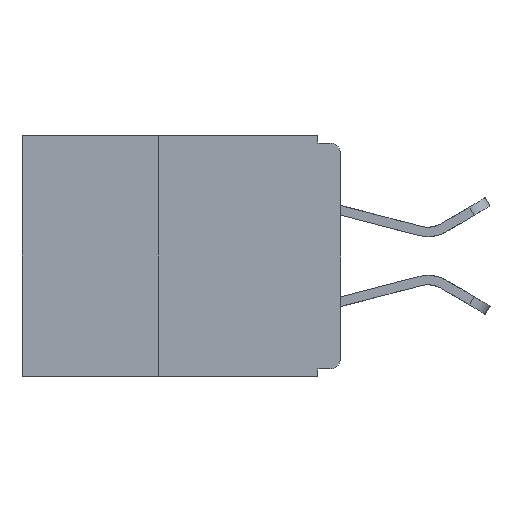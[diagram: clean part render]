
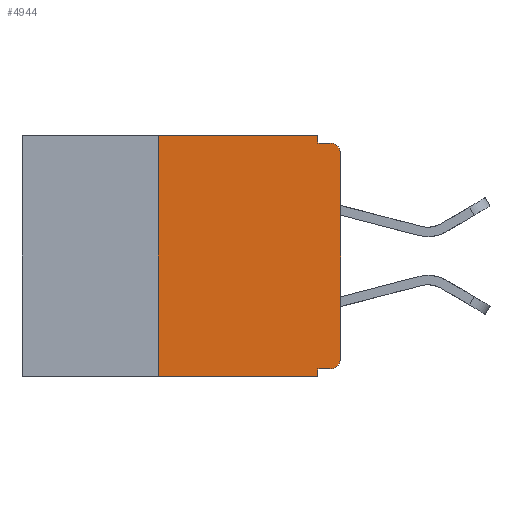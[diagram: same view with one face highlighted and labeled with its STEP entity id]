
A CAD part, left-side view. The second image highlights one B-rep face of the part: STEP entity #4944.
In plain terms, the highlighted planar face has unit normal (-1, 0, 0).
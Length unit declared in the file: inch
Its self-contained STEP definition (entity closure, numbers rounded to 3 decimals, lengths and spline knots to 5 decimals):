
#110 = VECTOR ( 'NONE', #1237, 39.37008 ) ;
#123 = VECTOR ( 'NONE', #5005, 39.37008 ) ;
#239 = VERTEX_POINT ( 'NONE', #5288 ) ;
#439 = DIRECTION ( 'NONE',  ( 0., 0., 1. ) ) ;
#592 = AXIS2_PLACEMENT_3D ( 'NONE', #5344, #15679, #6797 ) ;
#1014 = LINE ( 'NONE', #10217, #12454 ) ;
#1237 = DIRECTION ( 'NONE',  ( 0., 0., 1. ) ) ;
#1243 = DIRECTION ( 'NONE',  ( 0., 1., 0. ) ) ;
#1646 = VERTEX_POINT ( 'NONE', #3942 ) ;
#2058 = VECTOR ( 'NONE', #7723, 39.37008 ) ;
#2091 = DIRECTION ( 'NONE',  ( 0., 0., -1. ) ) ;
#2097 = DIRECTION ( 'NONE',  ( 1., 0., 0. ) ) ;
#2122 = PLANE ( 'NONE',  #6957 ) ;
#2150 = CIRCLE ( 'NONE', #592, 0.015 ) ;
#2185 = CARTESIAN_POINT ( 'NONE',  ( 0., 0.437, 0. ) ) ;
#2294 = CARTESIAN_POINT ( 'NONE',  ( 0., 0.437, 0. ) ) ;
#3084 = FACE_OUTER_BOUND ( 'NONE', #3452, .T. ) ;
#3151 = LINE ( 'NONE', #7966, #17905 ) ;
#3452 = EDGE_LOOP ( 'NONE', ( #7239, #8216, #10568, #11257, #12283, #12322, #14555, #15339, #15518, #17970 ) ) ;
#3489 = AXIS2_PLACEMENT_3D ( 'NONE', #4269, #14644, #5763 ) ;
#3777 = VECTOR ( 'NONE', #8352, 39.37008 ) ;
#3942 = CARTESIAN_POINT ( 'NONE',  ( 0., 0.25, -0.33 ) ) ;
#4077 = LINE ( 'NONE', #9123, #7091 ) ;
#4269 = CARTESIAN_POINT ( 'NONE',  ( 0., 0.015, -0.305 ) ) ;
#4428 = EDGE_CURVE ( 'NONE', #1646, #239, #4077, .T. ) ;
#4944 = ADVANCED_FACE ( 'NONE', ( #3084 ), #2122, .F. ) ;
#5005 = DIRECTION ( 'NONE',  ( 0., -1., 0. ) ) ;
#5288 = CARTESIAN_POINT ( 'NONE',  ( 0., 0.031, -0.33 ) ) ;
#5301 = VERTEX_POINT ( 'NONE', #13678 ) ;
#5344 = CARTESIAN_POINT ( 'NONE',  ( 0., 0.015, -0.025 ) ) ;
#5763 = DIRECTION ( 'NONE',  ( 0., 0., -1. ) ) ;
#5804 = VERTEX_POINT ( 'NONE', #18195 ) ;
#6047 = CARTESIAN_POINT ( 'NONE',  ( 0., 0.031, -0.33 ) ) ;
#6310 = CARTESIAN_POINT ( 'NONE',  ( 0., 0.015, -0.32 ) ) ;
#6580 = CARTESIAN_POINT ( 'NONE',  ( 0., 0.031, -0.01 ) ) ;
#6745 = EDGE_CURVE ( 'NONE', #11319, #8215, #17173, .T. ) ;
#6797 = DIRECTION ( 'NONE',  ( 0., 0., -1. ) ) ;
#6957 = AXIS2_PLACEMENT_3D ( 'NONE', #2185, #2097, #2091 ) ;
#7091 = VECTOR ( 'NONE', #9017, 39.37008 ) ;
#7239 = ORIENTED_EDGE ( 'NONE', *, *, #15188, .T. ) ;
#7723 = DIRECTION ( 'NONE',  ( 0., 0., -1. ) ) ;
#7748 = LINE ( 'NONE', #2294, #3777 ) ;
#7750 = CARTESIAN_POINT ( 'NONE',  ( 0., 0.031, 0. ) ) ;
#7966 = CARTESIAN_POINT ( 'NONE',  ( 0., 0., 0. ) ) ;
#8077 = VERTEX_POINT ( 'NONE', #6310 ) ;
#8215 = VERTEX_POINT ( 'NONE', #6580 ) ;
#8216 = ORIENTED_EDGE ( 'NONE', *, *, #16523, .T. ) ;
#8352 = DIRECTION ( 'NONE',  ( 0., -1., 0. ) ) ;
#9017 = DIRECTION ( 'NONE',  ( 0., -1., 0. ) ) ;
#9123 = CARTESIAN_POINT ( 'NONE',  ( 0., 0.437, -0.33 ) ) ;
#9588 = CARTESIAN_POINT ( 'NONE',  ( 0., 0., -0.025 ) ) ;
#10213 = CARTESIAN_POINT ( 'NONE',  ( 0., 0.25, -0.33 ) ) ;
#10217 = CARTESIAN_POINT ( 'NONE',  ( 0., 0., -0.32 ) ) ;
#10568 = ORIENTED_EDGE ( 'NONE', *, *, #12267, .F. ) ;
#10879 = EDGE_CURVE ( 'NONE', #5804, #239, #10991, .T. ) ;
#10991 = LINE ( 'NONE', #6047, #17400 ) ;
#11257 = ORIENTED_EDGE ( 'NONE', *, *, #6745, .F. ) ;
#11319 = VERTEX_POINT ( 'NONE', #14685 ) ;
#12085 = LINE ( 'NONE', #15337, #123 ) ;
#12267 = EDGE_CURVE ( 'NONE', #8215, #5301, #12085, .T. ) ;
#12283 = ORIENTED_EDGE ( 'NONE', *, *, #17419, .F. ) ;
#12322 = ORIENTED_EDGE ( 'NONE', *, *, #13229, .F. ) ;
#12454 = VECTOR ( 'NONE', #1243, 39.37008 ) ;
#12602 = EDGE_CURVE ( 'NONE', #8077, #16200, #17755, .T. ) ;
#13229 = EDGE_CURVE ( 'NONE', #1646, #18466, #15553, .T. ) ;
#13678 = CARTESIAN_POINT ( 'NONE',  ( 0., 0.015, -0.01 ) ) ;
#13728 = CARTESIAN_POINT ( 'NONE',  ( 0., 0.25, 0. ) ) ;
#14555 = ORIENTED_EDGE ( 'NONE', *, *, #4428, .T. ) ;
#14644 = DIRECTION ( 'NONE',  ( -1., 0., 0. ) ) ;
#14685 = CARTESIAN_POINT ( 'NONE',  ( 0., 0.031, 0. ) ) ;
#14954 = DIRECTION ( 'NONE',  ( 0., 0., -1. ) ) ;
#15188 = EDGE_CURVE ( 'NONE', #16200, #18582, #3151, .T. ) ;
#15337 = CARTESIAN_POINT ( 'NONE',  ( 0., 0., -0.01 ) ) ;
#15339 = ORIENTED_EDGE ( 'NONE', *, *, #10879, .F. ) ;
#15518 = ORIENTED_EDGE ( 'NONE', *, *, #15521, .F. ) ;
#15521 = EDGE_CURVE ( 'NONE', #8077, #5804, #1014, .T. ) ;
#15553 = LINE ( 'NONE', #10213, #110 ) ;
#15679 = DIRECTION ( 'NONE',  ( -1., 0., 0. ) ) ;
#16200 = VERTEX_POINT ( 'NONE', #17834 ) ;
#16523 = EDGE_CURVE ( 'NONE', #18582, #5301, #2150, .T. ) ;
#17173 = LINE ( 'NONE', #7750, #2058 ) ;
#17400 = VECTOR ( 'NONE', #14954, 39.37008 ) ;
#17419 = EDGE_CURVE ( 'NONE', #18466, #11319, #7748, .T. ) ;
#17755 = CIRCLE ( 'NONE', #3489, 0.015 ) ;
#17834 = CARTESIAN_POINT ( 'NONE',  ( 0., 0., -0.305 ) ) ;
#17905 = VECTOR ( 'NONE', #439, 39.37008 ) ;
#17970 = ORIENTED_EDGE ( 'NONE', *, *, #12602, .T. ) ;
#18195 = CARTESIAN_POINT ( 'NONE',  ( 0., 0.031, -0.32 ) ) ;
#18466 = VERTEX_POINT ( 'NONE', #13728 ) ;
#18582 = VERTEX_POINT ( 'NONE', #9588 ) ;
